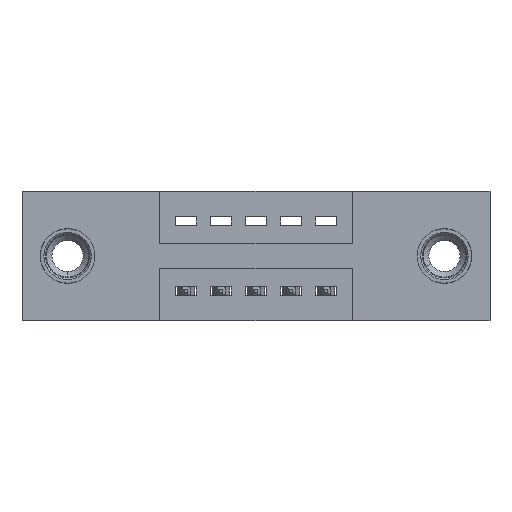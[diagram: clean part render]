
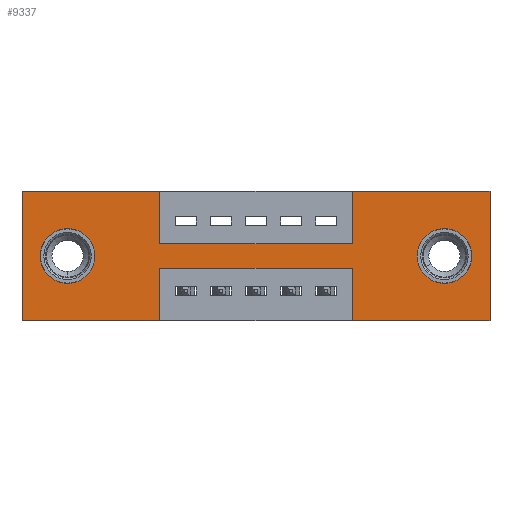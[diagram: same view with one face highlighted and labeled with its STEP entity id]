
A CAD part, front view. The second image highlights one B-rep face of the part: STEP entity #9337.
In plain terms, the highlighted planar face has unit normal (0, -1, 0).
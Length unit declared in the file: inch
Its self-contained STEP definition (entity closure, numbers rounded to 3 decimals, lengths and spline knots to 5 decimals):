
#1 = DIRECTION ( 'NONE',  ( 1., 0., 0. ) ) ;
#60 = VECTOR ( 'NONE', #4777, 39.37008 ) ;
#73 = ORIENTED_EDGE ( 'NONE', *, *, #7292, .F. ) ;
#200 = ORIENTED_EDGE ( 'NONE', *, *, #9310, .F. ) ;
#245 = DIRECTION ( 'NONE',  ( 0., 0., -1. ) ) ;
#270 = AXIS2_PLACEMENT_3D ( 'NONE', #7726, #3100, #8486 ) ;
#436 = CARTESIAN_POINT ( 'NONE',  ( 0.3925, 0., 0. ) ) ;
#469 = EDGE_CURVE ( 'NONE', #4981, #9891, #9550, .T. ) ;
#621 = LINE ( 'NONE', #4042, #8544 ) ;
#634 = CARTESIAN_POINT ( 'NONE',  ( 0.9425, 0., -0.37 ) ) ;
#680 = ORIENTED_EDGE ( 'NONE', *, *, #2016, .F. ) ;
#739 = DIRECTION ( 'NONE',  ( 0., 0., -1. ) ) ;
#899 = CARTESIAN_POINT ( 'NONE',  ( 0.9425, 0., 0. ) ) ;
#1072 = VERTEX_POINT ( 'NONE', #8292 ) ;
#1103 = CIRCLE ( 'NONE', #4118, 0.078 ) ;
#1200 = DIRECTION ( 'NONE',  ( 0., 0., -1. ) ) ;
#1314 = EDGE_CURVE ( 'NONE', #4625, #2426, #1103, .T. ) ;
#1353 = CARTESIAN_POINT ( 'NONE',  ( 0.3925, 0., 0. ) ) ;
#1421 = ORIENTED_EDGE ( 'NONE', *, *, #9727, .T. ) ;
#1470 = CARTESIAN_POINT ( 'NONE',  ( 1.335, 0., 0. ) ) ;
#1545 = VERTEX_POINT ( 'NONE', #1470 ) ;
#1602 = AXIS2_PLACEMENT_3D ( 'NONE', #9450, #4806, #245 ) ;
#1618 = VERTEX_POINT ( 'NONE', #9437 ) ;
#1961 = DIRECTION ( 'NONE',  ( 0., 0., -1. ) ) ;
#1981 = ORIENTED_EDGE ( 'NONE', *, *, #7887, .F. ) ;
#2016 = EDGE_CURVE ( 'NONE', #9891, #1545, #8184, .T. ) ;
#2177 = ORIENTED_EDGE ( 'NONE', *, *, #7215, .F. ) ;
#2181 = EDGE_CURVE ( 'NONE', #8914, #5751, #2876, .T. ) ;
#2199 = LINE ( 'NONE', #436, #8089 ) ;
#2249 = DIRECTION ( 'NONE',  ( 0., 1., 0. ) ) ;
#2290 = CARTESIAN_POINT ( 'NONE',  ( 0., 0., 0. ) ) ;
#2350 = VERTEX_POINT ( 'NONE', #1353 ) ;
#2426 = VERTEX_POINT ( 'NONE', #7618 ) ;
#2457 = ORIENTED_EDGE ( 'NONE', *, *, #2647, .F. ) ;
#2502 = DIRECTION ( 'NONE',  ( 1., 0., 0. ) ) ;
#2647 = EDGE_CURVE ( 'NONE', #5751, #6866, #621, .T. ) ;
#2687 = ORIENTED_EDGE ( 'NONE', *, *, #7949, .T. ) ;
#2723 = EDGE_CURVE ( 'NONE', #3054, #2350, #9642, .T. ) ;
#2754 = CARTESIAN_POINT ( 'NONE',  ( 0.3925, 0., -0.37 ) ) ;
#2876 = LINE ( 'NONE', #3410, #4424 ) ;
#3032 = DIRECTION ( 'NONE',  ( 0., 1., 0. ) ) ;
#3033 = CARTESIAN_POINT ( 'NONE',  ( 0.13, 0., -0.185 ) ) ;
#3054 = VERTEX_POINT ( 'NONE', #2290 ) ;
#3100 = DIRECTION ( 'NONE',  ( 0., 1., 0. ) ) ;
#3272 = VECTOR ( 'NONE', #3922, 39.37008 ) ;
#3327 = LINE ( 'NONE', #634, #8218 ) ;
#3361 = DIRECTION ( 'NONE',  ( 1., 0., 0. ) ) ;
#3388 = ORIENTED_EDGE ( 'NONE', *, *, #5521, .F. ) ;
#3392 = LINE ( 'NONE', #5311, #9324 ) ;
#3410 = CARTESIAN_POINT ( 'NONE',  ( 0.3925, 0., -0.37 ) ) ;
#3795 = DIRECTION ( 'NONE',  ( 0., 0., 1. ) ) ;
#3922 = DIRECTION ( 'NONE',  ( -1., 0., 0. ) ) ;
#3989 = CARTESIAN_POINT ( 'NONE',  ( 1.335, 0., 0. ) ) ;
#4042 = CARTESIAN_POINT ( 'NONE',  ( 0., 0., -0.37 ) ) ;
#4096 = LINE ( 'NONE', #3989, #60 ) ;
#4110 = ORIENTED_EDGE ( 'NONE', *, *, #1314, .T. ) ;
#4118 = AXIS2_PLACEMENT_3D ( 'NONE', #5954, #2249, #739 ) ;
#4397 = DIRECTION ( 'NONE',  ( 0., 0., 1. ) ) ;
#4424 = VECTOR ( 'NONE', #1961, 39.37008 ) ;
#4625 = VERTEX_POINT ( 'NONE', #5027 ) ;
#4777 = DIRECTION ( 'NONE',  ( 0., 0., -1. ) ) ;
#4806 = DIRECTION ( 'NONE',  ( 0., -1., 0. ) ) ;
#4981 = VERTEX_POINT ( 'NONE', #5447 ) ;
#5027 = CARTESIAN_POINT ( 'NONE',  ( 1.205, 0., -0.263 ) ) ;
#5311 = CARTESIAN_POINT ( 'NONE',  ( 0.3925, 0., -0.15 ) ) ;
#5425 = VECTOR ( 'NONE', #8723, 39.37008 ) ;
#5447 = CARTESIAN_POINT ( 'NONE',  ( 0.9425, 0., -0.15 ) ) ;
#5518 = VECTOR ( 'NONE', #3361, 39.37008 ) ;
#5521 = EDGE_CURVE ( 'NONE', #8861, #8914, #9202, .T. ) ;
#5612 = EDGE_LOOP ( 'NONE', ( #9313, #4110 ) ) ;
#5644 = CARTESIAN_POINT ( 'NONE',  ( 0., 0., 0. ) ) ;
#5751 = VERTEX_POINT ( 'NONE', #2754 ) ;
#5950 = VERTEX_POINT ( 'NONE', #7647 ) ;
#5954 = CARTESIAN_POINT ( 'NONE',  ( 1.205, 0., -0.185 ) ) ;
#6049 = CARTESIAN_POINT ( 'NONE',  ( 0., 0., 0. ) ) ;
#6182 = CIRCLE ( 'NONE', #8185, 0.078 ) ;
#6424 = LINE ( 'NONE', #6049, #8487 ) ;
#6866 = VERTEX_POINT ( 'NONE', #7114 ) ;
#6979 = CARTESIAN_POINT ( 'NONE',  ( 0.9425, 0., 0. ) ) ;
#7107 = CARTESIAN_POINT ( 'NONE',  ( 0.3925, 0., -0.15 ) ) ;
#7114 = CARTESIAN_POINT ( 'NONE',  ( 0., 0., -0.37 ) ) ;
#7144 = ORIENTED_EDGE ( 'NONE', *, *, #2181, .F. ) ;
#7215 = EDGE_CURVE ( 'NONE', #5950, #8861, #3327, .T. ) ;
#7292 = EDGE_CURVE ( 'NONE', #8606, #4981, #3392, .T. ) ;
#7321 = CARTESIAN_POINT ( 'NONE',  ( 0.3925, 0., -0.22 ) ) ;
#7389 = ORIENTED_EDGE ( 'NONE', *, *, #2723, .F. ) ;
#7454 = VERTEX_POINT ( 'NONE', #7878 ) ;
#7618 = CARTESIAN_POINT ( 'NONE',  ( 1.205, 0., -0.107 ) ) ;
#7626 = DIRECTION ( 'NONE',  ( 0., 0., 1. ) ) ;
#7647 = CARTESIAN_POINT ( 'NONE',  ( 0.9425, 0., -0.37 ) ) ;
#7663 = CARTESIAN_POINT ( 'NONE',  ( 1.205, 0., -0.185 ) ) ;
#7726 = CARTESIAN_POINT ( 'NONE',  ( 0.13, 0., -0.185 ) ) ;
#7772 = CIRCLE ( 'NONE', #270, 0.078 ) ;
#7789 = ORIENTED_EDGE ( 'NONE', *, *, #9855, .F. ) ;
#7878 = CARTESIAN_POINT ( 'NONE',  ( 0.13, 0., -0.263 ) ) ;
#7887 = EDGE_CURVE ( 'NONE', #6866, #3054, #6424, .T. ) ;
#7894 = PLANE ( 'NONE',  #1602 ) ;
#7908 = EDGE_CURVE ( 'NONE', #2426, #4625, #6182, .T. ) ;
#7947 = VECTOR ( 'NONE', #2502, 39.37008 ) ;
#7949 = EDGE_CURVE ( 'NONE', #1618, #7454, #7772, .T. ) ;
#7976 = FACE_BOUND ( 'NONE', #5612, .T. ) ;
#8089 = VECTOR ( 'NONE', #1200, 39.37008 ) ;
#8112 = AXIS2_PLACEMENT_3D ( 'NONE', #3033, #8424, #3795 ) ;
#8184 = LINE ( 'NONE', #9407, #7947 ) ;
#8185 = AXIS2_PLACEMENT_3D ( 'NONE', #7663, #3032, #8422 ) ;
#8209 = CIRCLE ( 'NONE', #8112, 0.078 ) ;
#8217 = FACE_BOUND ( 'NONE', #8761, .T. ) ;
#8218 = VECTOR ( 'NONE', #4397, 39.37008 ) ;
#8292 = CARTESIAN_POINT ( 'NONE',  ( 1.335, 0., -0.37 ) ) ;
#8422 = DIRECTION ( 'NONE',  ( 0., 0., -1. ) ) ;
#8424 = DIRECTION ( 'NONE',  ( 0., 1., 0. ) ) ;
#8486 = DIRECTION ( 'NONE',  ( 0., 0., 1. ) ) ;
#8487 = VECTOR ( 'NONE', #7626, 39.37008 ) ;
#8544 = VECTOR ( 'NONE', #8670, 39.37008 ) ;
#8553 = CARTESIAN_POINT ( 'NONE',  ( 0., 0., -0.37 ) ) ;
#8606 = VERTEX_POINT ( 'NONE', #7107 ) ;
#8670 = DIRECTION ( 'NONE',  ( -1., 0., 0. ) ) ;
#8702 = ORIENTED_EDGE ( 'NONE', *, *, #9508, .F. ) ;
#8723 = DIRECTION ( 'NONE',  ( 0., 0., 1. ) ) ;
#8761 = EDGE_LOOP ( 'NONE', ( #2687, #1421 ) ) ;
#8861 = VERTEX_POINT ( 'NONE', #9560 ) ;
#8914 = VERTEX_POINT ( 'NONE', #7321 ) ;
#9202 = LINE ( 'NONE', #9325, #3272 ) ;
#9290 = VECTOR ( 'NONE', #9331, 39.37008 ) ;
#9310 = EDGE_CURVE ( 'NONE', #1545, #1072, #4096, .T. ) ;
#9311 = ORIENTED_EDGE ( 'NONE', *, *, #469, .F. ) ;
#9313 = ORIENTED_EDGE ( 'NONE', *, *, #7908, .T. ) ;
#9324 = VECTOR ( 'NONE', #1, 39.37008 ) ;
#9325 = CARTESIAN_POINT ( 'NONE',  ( 0.3925, 0., -0.22 ) ) ;
#9331 = DIRECTION ( 'NONE',  ( -1., 0., 0. ) ) ;
#9337 = ADVANCED_FACE ( 'NONE', ( #7976, #8217, #9793 ), #7894, .T. ) ;
#9407 = CARTESIAN_POINT ( 'NONE',  ( 0., 0., 0. ) ) ;
#9437 = CARTESIAN_POINT ( 'NONE',  ( 0.13, 0., -0.107 ) ) ;
#9450 = CARTESIAN_POINT ( 'NONE',  ( 0., 0., -0.37 ) ) ;
#9508 = EDGE_CURVE ( 'NONE', #2350, #8606, #2199, .T. ) ;
#9550 = LINE ( 'NONE', #6979, #5425 ) ;
#9560 = CARTESIAN_POINT ( 'NONE',  ( 0.9425, 0., -0.22 ) ) ;
#9642 = LINE ( 'NONE', #5644, #5518 ) ;
#9697 = EDGE_LOOP ( 'NONE', ( #7144, #3388, #2177, #7789, #200, #680, #9311, #73, #8702, #7389, #1981, #2457 ) ) ;
#9727 = EDGE_CURVE ( 'NONE', #7454, #1618, #8209, .T. ) ;
#9785 = LINE ( 'NONE', #8553, #9290 ) ;
#9793 = FACE_OUTER_BOUND ( 'NONE', #9697, .T. ) ;
#9855 = EDGE_CURVE ( 'NONE', #1072, #5950, #9785, .T. ) ;
#9891 = VERTEX_POINT ( 'NONE', #899 ) ;
